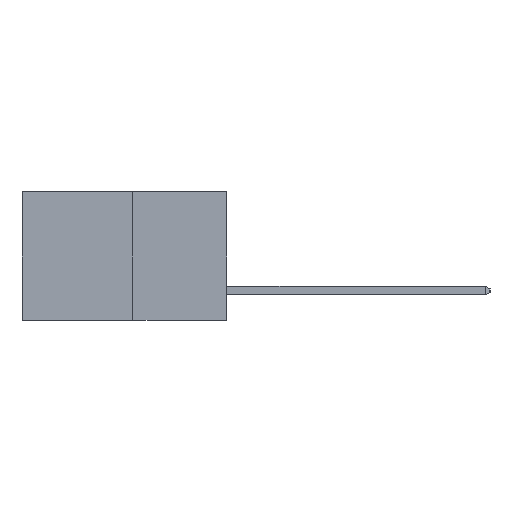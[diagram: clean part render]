
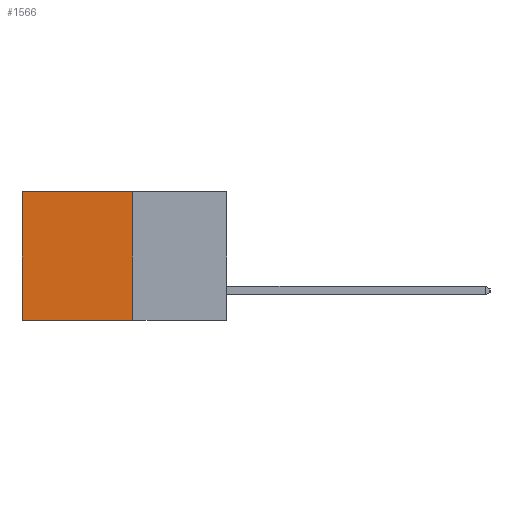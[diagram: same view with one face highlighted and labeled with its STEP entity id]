
A CAD part, left-side view. The second image highlights one B-rep face of the part: STEP entity #1566.
In plain terms, the highlighted planar face has unit normal (-1, 0, 0).
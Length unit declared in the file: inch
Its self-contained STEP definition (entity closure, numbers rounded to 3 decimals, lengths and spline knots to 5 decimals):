
#1566 = ADVANCED_FACE ( 'NONE', ( #20846 ), #8028, .F. ) ;
#1650 = DIRECTION ( 'NONE',  ( 0., 0., -1. ) ) ;
#1745 = CARTESIAN_POINT ( 'NONE',  ( 0.277, 0.27, 0. ) ) ;
#1785 = VECTOR ( 'NONE', #8655, 39.37008 ) ;
#2068 = VERTEX_POINT ( 'NONE', #1745 ) ;
#2165 = VERTEX_POINT ( 'NONE', #4021 ) ;
#2684 = EDGE_CURVE ( 'NONE', #2068, #5297, #11241, .T. ) ;
#2689 = DIRECTION ( 'NONE',  ( 0., 0., -1. ) ) ;
#4021 = CARTESIAN_POINT ( 'NONE',  ( 0.277, 0.59, -0.37 ) ) ;
#4980 = CARTESIAN_POINT ( 'NONE',  ( 0.277, 0.27, 0. ) ) ;
#5297 = VERTEX_POINT ( 'NONE', #16571 ) ;
#5439 = VECTOR ( 'NONE', #12095, 39.37008 ) ;
#5920 = CARTESIAN_POINT ( 'NONE',  ( 0.277, 0.27, -0.37 ) ) ;
#7746 = VECTOR ( 'NONE', #13114, 39.37008 ) ;
#8028 = PLANE ( 'NONE',  #16187 ) ;
#8529 = CARTESIAN_POINT ( 'NONE',  ( 0.277, 0.27, -0.37 ) ) ;
#8655 = DIRECTION ( 'NONE',  ( 0., 0., -1. ) ) ;
#8840 = VECTOR ( 'NONE', #1650, 39.37008 ) ;
#9700 = ORIENTED_EDGE ( 'NONE', *, *, #12881, .T. ) ;
#10639 = EDGE_CURVE ( 'NONE', #5297, #2165, #12516, .T. ) ;
#11018 = CARTESIAN_POINT ( 'NONE',  ( 0.277, 0.59, 0. ) ) ;
#11031 = EDGE_CURVE ( 'NONE', #22628, #2165, #18215, .T. ) ;
#11241 = LINE ( 'NONE', #8529, #1785 ) ;
#12095 = DIRECTION ( 'NONE',  ( 0., 1., 0. ) ) ;
#12516 = LINE ( 'NONE', #5920, #7746 ) ;
#12881 = EDGE_CURVE ( 'NONE', #2068, #22628, #17359, .T. ) ;
#13114 = DIRECTION ( 'NONE',  ( 0., 1., 0. ) ) ;
#14493 = EDGE_LOOP ( 'NONE', ( #18170, #15633, #18877, #9700 ) ) ;
#15633 = ORIENTED_EDGE ( 'NONE', *, *, #10639, .F. ) ;
#16187 = AXIS2_PLACEMENT_3D ( 'NONE', #21618, #18014, #2689 ) ;
#16571 = CARTESIAN_POINT ( 'NONE',  ( 0.277, 0.27, -0.37 ) ) ;
#17359 = LINE ( 'NONE', #4980, #5439 ) ;
#18014 = DIRECTION ( 'NONE',  ( 1., 0., 0. ) ) ;
#18170 = ORIENTED_EDGE ( 'NONE', *, *, #11031, .T. ) ;
#18215 = LINE ( 'NONE', #22663, #8840 ) ;
#18877 = ORIENTED_EDGE ( 'NONE', *, *, #2684, .F. ) ;
#20846 = FACE_OUTER_BOUND ( 'NONE', #14493, .T. ) ;
#21618 = CARTESIAN_POINT ( 'NONE',  ( 0.277, 0.27, -0.37 ) ) ;
#22628 = VERTEX_POINT ( 'NONE', #11018 ) ;
#22663 = CARTESIAN_POINT ( 'NONE',  ( 0.277, 0.59, -0.37 ) ) ;
